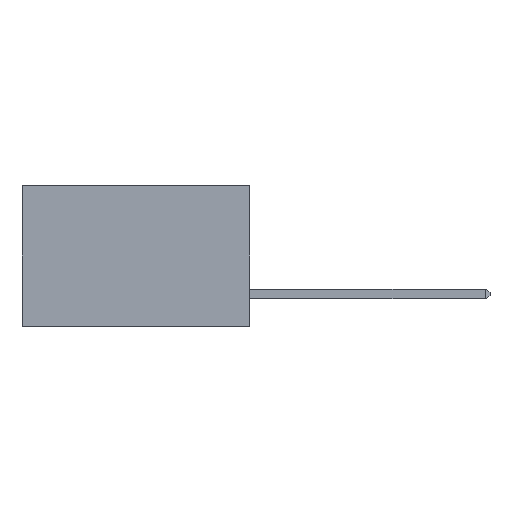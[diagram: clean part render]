
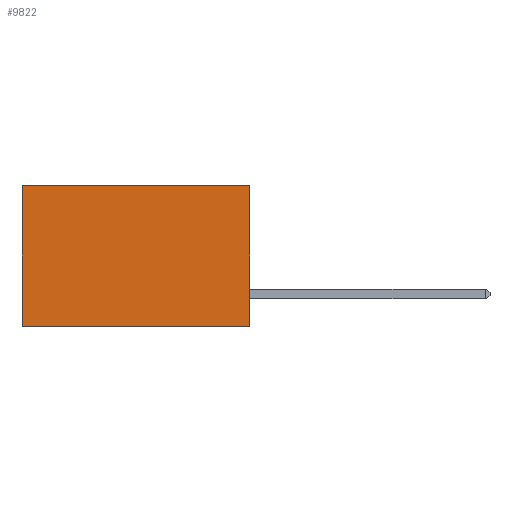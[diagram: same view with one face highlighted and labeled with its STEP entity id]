
A CAD part, left-side view. The second image highlights one B-rep face of the part: STEP entity #9822.
In plain terms, the highlighted planar face has unit normal (-1, 0, 0).
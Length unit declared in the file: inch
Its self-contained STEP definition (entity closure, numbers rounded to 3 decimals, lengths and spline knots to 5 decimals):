
#1060 = CARTESIAN_POINT ( 'NONE',  ( 0.2875, 0., 0. ) ) ;
#1787 = VECTOR ( 'NONE', #12830, 39.37008 ) ;
#2624 = LINE ( 'NONE', #13551, #34032 ) ;
#2862 = DIRECTION ( 'NONE',  ( 0., 1., 0. ) ) ;
#7205 = CARTESIAN_POINT ( 'NONE',  ( 0.2875, 0., -0.37 ) ) ;
#8043 = VERTEX_POINT ( 'NONE', #36822 ) ;
#9117 = EDGE_LOOP ( 'NONE', ( #23153, #32214, #15313, #22433 ) ) ;
#9822 = ADVANCED_FACE ( 'NONE', ( #28030 ), #10306, .F. ) ;
#10306 = PLANE ( 'NONE',  #28440 ) ;
#11794 = VECTOR ( 'NONE', #2862, 39.37008 ) ;
#12033 = VERTEX_POINT ( 'NONE', #39978 ) ;
#12305 = VERTEX_POINT ( 'NONE', #16348 ) ;
#12830 = DIRECTION ( 'NONE',  ( 0., 0., -1. ) ) ;
#13074 = VECTOR ( 'NONE', #29459, 39.37008 ) ;
#13551 = CARTESIAN_POINT ( 'NONE',  ( 0.2875, 0., 0. ) ) ;
#14068 = LINE ( 'NONE', #1060, #13074 ) ;
#15313 = ORIENTED_EDGE ( 'NONE', *, *, #31407, .F. ) ;
#16348 = CARTESIAN_POINT ( 'NONE',  ( 0.2875, 0.6, -0.37 ) ) ;
#16592 = DIRECTION ( 'NONE',  ( 1., 0., 0. ) ) ;
#18575 = VERTEX_POINT ( 'NONE', #7205 ) ;
#20255 = EDGE_CURVE ( 'NONE', #8043, #12033, #14068, .T. ) ;
#22433 = ORIENTED_EDGE ( 'NONE', *, *, #20255, .T. ) ;
#23153 = ORIENTED_EDGE ( 'NONE', *, *, #39129, .T. ) ;
#23767 = DIRECTION ( 'NONE',  ( 0., 0., -1. ) ) ;
#25379 = CARTESIAN_POINT ( 'NONE',  ( 0.2875, 0.6, 0. ) ) ;
#26983 = LINE ( 'NONE', #25379, #1787 ) ;
#28030 = FACE_OUTER_BOUND ( 'NONE', #9117, .T. ) ;
#28440 = AXIS2_PLACEMENT_3D ( 'NONE', #35239, #16592, #38318 ) ;
#29459 = DIRECTION ( 'NONE',  ( 0., 1., 0. ) ) ;
#31407 = EDGE_CURVE ( 'NONE', #8043, #18575, #2624, .T. ) ;
#32214 = ORIENTED_EDGE ( 'NONE', *, *, #40390, .F. ) ;
#34032 = VECTOR ( 'NONE', #23767, 39.37008 ) ;
#35239 = CARTESIAN_POINT ( 'NONE',  ( 0.2875, 0., 0. ) ) ;
#36644 = LINE ( 'NONE', #40313, #11794 ) ;
#36822 = CARTESIAN_POINT ( 'NONE',  ( 0.2875, 0., 0. ) ) ;
#38318 = DIRECTION ( 'NONE',  ( 0., 0., -1. ) ) ;
#39129 = EDGE_CURVE ( 'NONE', #12033, #12305, #26983, .T. ) ;
#39978 = CARTESIAN_POINT ( 'NONE',  ( 0.2875, 0.6, 0. ) ) ;
#40313 = CARTESIAN_POINT ( 'NONE',  ( 0.2875, 0., -0.37 ) ) ;
#40390 = EDGE_CURVE ( 'NONE', #18575, #12305, #36644, .T. ) ;
